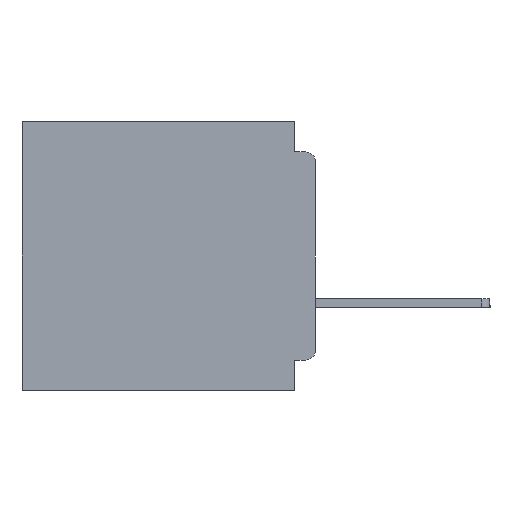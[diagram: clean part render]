
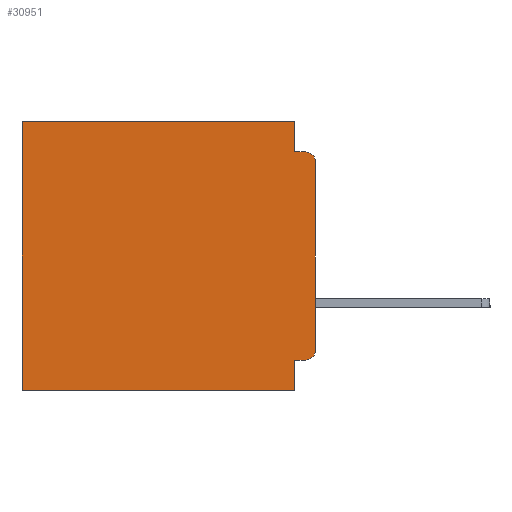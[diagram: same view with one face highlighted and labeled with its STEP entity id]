
A CAD part, left-side view. The second image highlights one B-rep face of the part: STEP entity #30951.
In plain terms, the highlighted planar face has unit normal (-1, 0, 0).
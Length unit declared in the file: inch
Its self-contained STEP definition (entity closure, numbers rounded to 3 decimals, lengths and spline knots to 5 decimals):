
#250 = VECTOR ( 'NONE', #36769, 39.37008 ) ;
#1253 = EDGE_LOOP ( 'NONE', ( #4869, #3943, #18822, #35303, #10356, #22756, #33174, #3278, #8467, #38656 ) ) ;
#1348 = VERTEX_POINT ( 'NONE', #35313 ) ;
#2124 = CARTESIAN_POINT ( 'NONE',  ( 0.3, 0.015, -0.355 ) ) ;
#2596 = CARTESIAN_POINT ( 'NONE',  ( 0.3, 0.437, -0.4 ) ) ;
#2768 = EDGE_CURVE ( 'NONE', #22523, #22129, #35640, .T. ) ;
#3278 = ORIENTED_EDGE ( 'NONE', *, *, #30884, .F. ) ;
#3329 = DIRECTION ( 'NONE',  ( -1., 0., 0. ) ) ;
#3943 = ORIENTED_EDGE ( 'NONE', *, *, #18116, .T. ) ;
#4170 = DIRECTION ( 'NONE',  ( 0., 1., 0. ) ) ;
#4225 = VERTEX_POINT ( 'NONE', #32997 ) ;
#4520 = CARTESIAN_POINT ( 'NONE',  ( 0.3, 0.031, 0. ) ) ;
#4869 = ORIENTED_EDGE ( 'NONE', *, *, #30293, .F. ) ;
#5749 = PLANE ( 'NONE',  #37122 ) ;
#6225 = LINE ( 'NONE', #18008, #38809 ) ;
#6810 = EDGE_CURVE ( 'NONE', #4225, #36079, #6225, .T. ) ;
#6872 = CARTESIAN_POINT ( 'NONE',  ( 0.3, 0., -0.4 ) ) ;
#7260 = VECTOR ( 'NONE', #20750, 39.37008 ) ;
#7459 = CIRCLE ( 'NONE', #10558, 0.015 ) ;
#7508 = LINE ( 'NONE', #12268, #250 ) ;
#8467 = ORIENTED_EDGE ( 'NONE', *, *, #2768, .F. ) ;
#8854 = DIRECTION ( 'NONE',  ( 1., 0., 0. ) ) ;
#9833 = EDGE_CURVE ( 'NONE', #22523, #32639, #7459, .T. ) ;
#10243 = CIRCLE ( 'NONE', #24322, 0.015 ) ;
#10356 = ORIENTED_EDGE ( 'NONE', *, *, #20955, .T. ) ;
#10558 = AXIS2_PLACEMENT_3D ( 'NONE', #21833, #3329, #24857 ) ;
#11536 = CARTESIAN_POINT ( 'NONE',  ( 0.3, 0., -0.34 ) ) ;
#11682 = CARTESIAN_POINT ( 'NONE',  ( 0.3, 0.031, 0. ) ) ;
#12268 = CARTESIAN_POINT ( 'NONE',  ( 0.3, 0., 0. ) ) ;
#12517 = CARTESIAN_POINT ( 'NONE',  ( 0.3, 0.031, -0.355 ) ) ;
#13013 = DIRECTION ( 'NONE',  ( 0., 0., -1. ) ) ;
#13112 = VECTOR ( 'NONE', #24164, 39.37008 ) ;
#13404 = VECTOR ( 'NONE', #13013, 39.37008 ) ;
#14735 = DIRECTION ( 'NONE',  ( 0., 0., -1. ) ) ;
#14874 = VERTEX_POINT ( 'NONE', #22197 ) ;
#16042 = DIRECTION ( 'NONE',  ( 0., -1., 0. ) ) ;
#16464 = CARTESIAN_POINT ( 'NONE',  ( 0.3, 0.015, -0.06 ) ) ;
#16909 = LINE ( 'NONE', #37454, #25127 ) ;
#17619 = CARTESIAN_POINT ( 'NONE',  ( 0.3, 0.437, 0. ) ) ;
#18008 = CARTESIAN_POINT ( 'NONE',  ( 0.3, 0., -0.4 ) ) ;
#18116 = EDGE_CURVE ( 'NONE', #1348, #14874, #10243, .T. ) ;
#18209 = VERTEX_POINT ( 'NONE', #4520 ) ;
#18427 = CARTESIAN_POINT ( 'NONE',  ( 0.3, 0.437, -0.4 ) ) ;
#18645 = DIRECTION ( 'NONE',  ( 0., 1., 0. ) ) ;
#18822 = ORIENTED_EDGE ( 'NONE', *, *, #29607, .F. ) ;
#19442 = VECTOR ( 'NONE', #4170, 39.37008 ) ;
#19616 = DIRECTION ( 'NONE',  ( 0., 0., -1. ) ) ;
#19726 = VECTOR ( 'NONE', #14735, 39.37008 ) ;
#20750 = DIRECTION ( 'NONE',  ( 0., 0., -1. ) ) ;
#20955 = EDGE_CURVE ( 'NONE', #18209, #35586, #7508, .T. ) ;
#21833 = CARTESIAN_POINT ( 'NONE',  ( 0.3, 0.015, -0.34 ) ) ;
#22129 = VERTEX_POINT ( 'NONE', #12517 ) ;
#22197 = CARTESIAN_POINT ( 'NONE',  ( 0.3, 0.015, -0.045 ) ) ;
#22523 = VERTEX_POINT ( 'NONE', #2124 ) ;
#22728 = FACE_OUTER_BOUND ( 'NONE', #1253, .T. ) ;
#22756 = ORIENTED_EDGE ( 'NONE', *, *, #36573, .T. ) ;
#24164 = DIRECTION ( 'NONE',  ( 0., 0., -1. ) ) ;
#24322 = AXIS2_PLACEMENT_3D ( 'NONE', #16464, #37881, #19616 ) ;
#24599 = LINE ( 'NONE', #6872, #13404 ) ;
#24857 = DIRECTION ( 'NONE',  ( 0., 0., -1. ) ) ;
#25127 = VECTOR ( 'NONE', #16042, 39.37008 ) ;
#26382 = VERTEX_POINT ( 'NONE', #38397 ) ;
#27258 = CARTESIAN_POINT ( 'NONE',  ( 0.3, 0., -0.4 ) ) ;
#27841 = LINE ( 'NONE', #11682, #19726 ) ;
#28519 = LINE ( 'NONE', #2596, #13112 ) ;
#29607 = EDGE_CURVE ( 'NONE', #26382, #14874, #16909, .T. ) ;
#29779 = CARTESIAN_POINT ( 'NONE',  ( 0.3, 0.031, -0.4 ) ) ;
#30293 = EDGE_CURVE ( 'NONE', #1348, #32639, #24599, .T. ) ;
#30297 = DIRECTION ( 'NONE',  ( 0., 0., -1. ) ) ;
#30884 = EDGE_CURVE ( 'NONE', #22129, #4225, #31740, .T. ) ;
#30951 = ADVANCED_FACE ( 'NONE', ( #22728 ), #5749, .F. ) ;
#31740 = LINE ( 'NONE', #29779, #7260 ) ;
#32639 = VERTEX_POINT ( 'NONE', #11536 ) ;
#32997 = CARTESIAN_POINT ( 'NONE',  ( 0.3, 0.031, -0.4 ) ) ;
#33174 = ORIENTED_EDGE ( 'NONE', *, *, #6810, .F. ) ;
#35303 = ORIENTED_EDGE ( 'NONE', *, *, #39608, .F. ) ;
#35313 = CARTESIAN_POINT ( 'NONE',  ( 0.3, 0., -0.06 ) ) ;
#35586 = VERTEX_POINT ( 'NONE', #17619 ) ;
#35640 = LINE ( 'NONE', #39036, #19442 ) ;
#36079 = VERTEX_POINT ( 'NONE', #18427 ) ;
#36573 = EDGE_CURVE ( 'NONE', #35586, #36079, #28519, .T. ) ;
#36769 = DIRECTION ( 'NONE',  ( 0., 1., 0. ) ) ;
#37122 = AXIS2_PLACEMENT_3D ( 'NONE', #27258, #8854, #30297 ) ;
#37454 = CARTESIAN_POINT ( 'NONE',  ( 0.3, 0., -0.045 ) ) ;
#37881 = DIRECTION ( 'NONE',  ( -1., 0., 0. ) ) ;
#38397 = CARTESIAN_POINT ( 'NONE',  ( 0.3, 0.031, -0.045 ) ) ;
#38656 = ORIENTED_EDGE ( 'NONE', *, *, #9833, .T. ) ;
#38809 = VECTOR ( 'NONE', #18645, 39.37008 ) ;
#39036 = CARTESIAN_POINT ( 'NONE',  ( 0.3, 0., -0.355 ) ) ;
#39608 = EDGE_CURVE ( 'NONE', #18209, #26382, #27841, .T. ) ;
